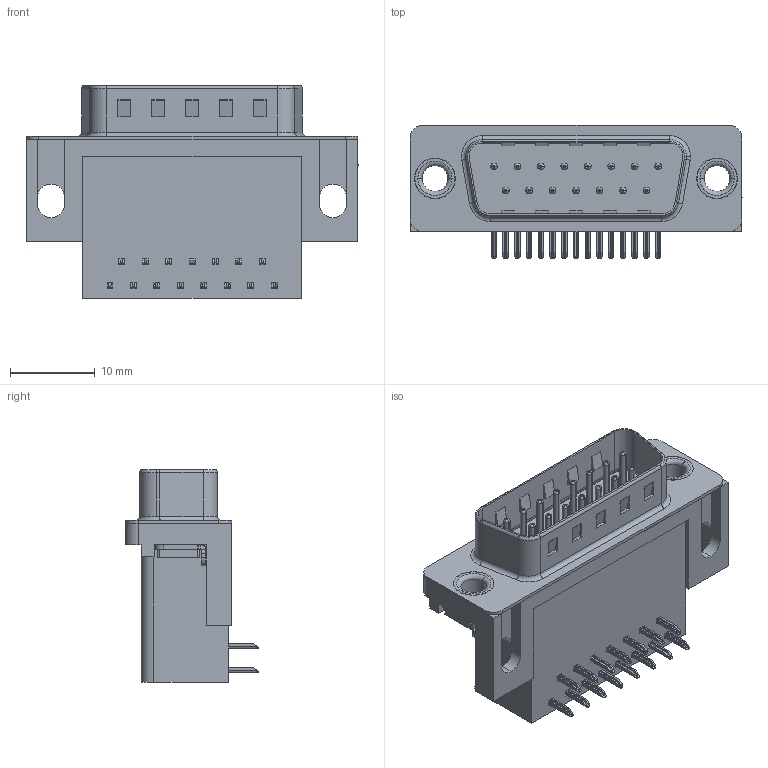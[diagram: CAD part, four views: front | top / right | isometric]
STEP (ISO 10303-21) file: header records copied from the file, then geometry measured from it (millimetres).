
FILE_DESCRIPTION (( 'STEP AP203' ), '1' );
FILE_NAME ('625-015-262-001.STEP', '2018-11-05T22:15:37', ( '' ), ( '' ), 'SwSTEP 2.0', 'SolidWorks 2016', '' );
FILE_SCHEMA (( 'CONFIG_CONTROL_DESIGN' ));
Length unit declared in the file: millimetre
Products named in the file (7): 625 Shell_15 Socket; 625 Non Board Mount; 625 Contact Bottom; 625 Thru Hole Rivet; 625 Housing_15 Socket; 625 Contact Top; 625-015-262-001
Assembly tree (21 placements, depth 2):
  625-015-262-001
    625 Housing_15 Socket
    625 Shell_15 Socket
    625 Contact Bottom  x7
    625 Contact Top  x8
    625 Non Board Mount  x2
    625 Thru Hole Rivet  x2
Bounding box: 39.22 x 15.73 x 25.16 mm (x, y, z)
Volume: 6203 mm3; surface area: 6267 mm2
Topology: 21 solids, 21 shells, 1437 faces, 3565 edges, 2207 vertices
Faces by surface type: plane 895, cylinder 425, torus 117
Entity records: 16681 total; most frequent: DIRECTION 2756, CARTESIAN_POINT 2701, ORIENTED_EDGE 2600, EDGE_CURVE 1300, AXIS2_PLACEMENT_3D 924, VECTOR 908, LINE 908, VERTEX_POINT 829
